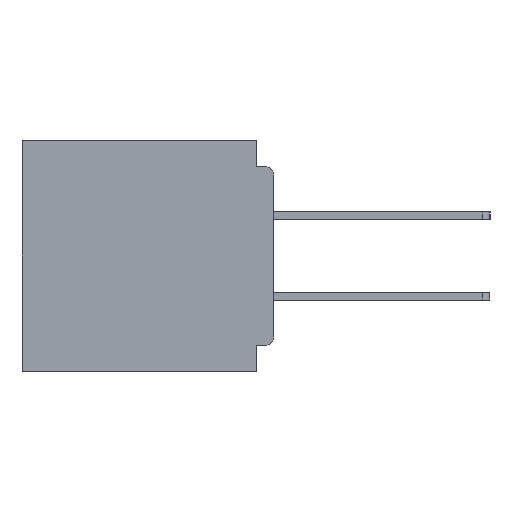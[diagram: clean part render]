
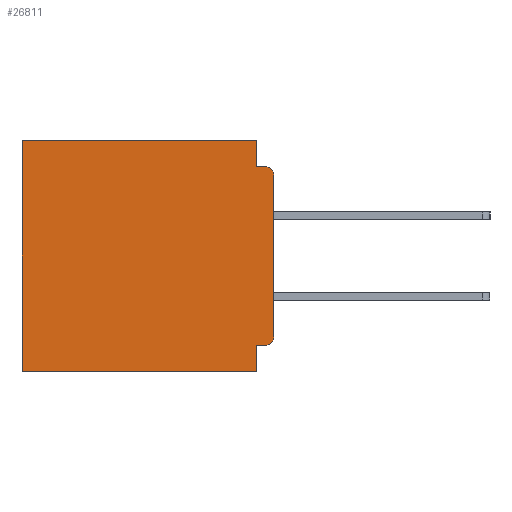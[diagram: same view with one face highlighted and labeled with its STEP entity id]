
A CAD part, left-side view. The second image highlights one B-rep face of the part: STEP entity #26811.
In plain terms, the highlighted planar face has unit normal (-1, 0, 0).
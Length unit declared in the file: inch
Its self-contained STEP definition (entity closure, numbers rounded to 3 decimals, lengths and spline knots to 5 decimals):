
#388 = CARTESIAN_POINT ( 'NONE',  ( 0.3, 0.031, 0. ) ) ;
#550 = CARTESIAN_POINT ( 'NONE',  ( 0.3, 0., -0.4 ) ) ;
#1070 = ORIENTED_EDGE ( 'NONE', *, *, #37587, .T. ) ;
#2581 = ORIENTED_EDGE ( 'NONE', *, *, #10394, .F. ) ;
#2887 = LINE ( 'NONE', #26888, #10167 ) ;
#3067 = ORIENTED_EDGE ( 'NONE', *, *, #6784, .F. ) ;
#3721 = DIRECTION ( 'NONE',  ( 1., 0., 0. ) ) ;
#3851 = CARTESIAN_POINT ( 'NONE',  ( 0.3, 0.437, 0. ) ) ;
#3932 = VECTOR ( 'NONE', #30655, 39.37008 ) ;
#4129 = VERTEX_POINT ( 'NONE', #21061 ) ;
#4271 = EDGE_CURVE ( 'NONE', #32339, #22659, #35562, .T. ) ;
#4812 = CARTESIAN_POINT ( 'NONE',  ( 0.3, 0., -0.045 ) ) ;
#4949 = VERTEX_POINT ( 'NONE', #7442 ) ;
#5126 = CARTESIAN_POINT ( 'NONE',  ( 0.3, 0., 0. ) ) ;
#5230 = ORIENTED_EDGE ( 'NONE', *, *, #27300, .T. ) ;
#5652 = AXIS2_PLACEMENT_3D ( 'NONE', #24552, #6122, #27612 ) ;
#6122 = DIRECTION ( 'NONE',  ( -1., 0., 0. ) ) ;
#6219 = AXIS2_PLACEMENT_3D ( 'NONE', #30311, #11955, #33346 ) ;
#6582 = EDGE_CURVE ( 'NONE', #6972, #24059, #34110, .T. ) ;
#6784 = EDGE_CURVE ( 'NONE', #4949, #7276, #2887, .T. ) ;
#6972 = VERTEX_POINT ( 'NONE', #37114 ) ;
#7069 = CIRCLE ( 'NONE', #5652, 0.015 ) ;
#7276 = VERTEX_POINT ( 'NONE', #20208 ) ;
#7338 = ORIENTED_EDGE ( 'NONE', *, *, #4271, .T. ) ;
#7442 = CARTESIAN_POINT ( 'NONE',  ( 0.3, 0., -0.06 ) ) ;
#7525 = VECTOR ( 'NONE', #17729, 39.37008 ) ;
#7939 = DIRECTION ( 'NONE',  ( 0., -1., 0. ) ) ;
#8235 = ORIENTED_EDGE ( 'NONE', *, *, #6582, .F. ) ;
#8476 = VECTOR ( 'NONE', #7939, 39.37008 ) ;
#8513 = DIRECTION ( 'NONE',  ( 0., 0., -1. ) ) ;
#9272 = AXIS2_PLACEMENT_3D ( 'NONE', #550, #3721, #25249 ) ;
#9529 = CARTESIAN_POINT ( 'NONE',  ( 0.3, 0., -0.355 ) ) ;
#9587 = DIRECTION ( 'NONE',  ( 0., 0., -1. ) ) ;
#9602 = DIRECTION ( 'NONE',  ( 0., 1., 0. ) ) ;
#10167 = VECTOR ( 'NONE', #8513, 39.37008 ) ;
#10394 = EDGE_CURVE ( 'NONE', #36185, #4129, #24817, .T. ) ;
#10654 = VECTOR ( 'NONE', #29050, 39.37008 ) ;
#10665 = CARTESIAN_POINT ( 'NONE',  ( 0.3, 0.031, -0.4 ) ) ;
#11060 = CARTESIAN_POINT ( 'NONE',  ( 0.3, 0.031, -0.045 ) ) ;
#11415 = VERTEX_POINT ( 'NONE', #19055 ) ;
#11955 = DIRECTION ( 'NONE',  ( -1., 0., 0. ) ) ;
#12642 = DIRECTION ( 'NONE',  ( 0., 1., 0. ) ) ;
#12703 = CARTESIAN_POINT ( 'NONE',  ( 0.3, 0.437, -0.4 ) ) ;
#14266 = ORIENTED_EDGE ( 'NONE', *, *, #19212, .F. ) ;
#15522 = CARTESIAN_POINT ( 'NONE',  ( 0.3, 0.031, -0.4 ) ) ;
#15609 = EDGE_CURVE ( 'NONE', #32339, #36185, #31038, .T. ) ;
#15971 = ORIENTED_EDGE ( 'NONE', *, *, #29117, .T. ) ;
#16676 = ORIENTED_EDGE ( 'NONE', *, *, #15609, .F. ) ;
#17729 = DIRECTION ( 'NONE',  ( 0., 0., -1. ) ) ;
#18768 = CARTESIAN_POINT ( 'NONE',  ( 0.3, 0.437, -0.4 ) ) ;
#18920 = CARTESIAN_POINT ( 'NONE',  ( 0.3, 0., -0.4 ) ) ;
#19055 = CARTESIAN_POINT ( 'NONE',  ( 0.3, 0.015, -0.355 ) ) ;
#19136 = PLANE ( 'NONE',  #9272 ) ;
#19212 = EDGE_CURVE ( 'NONE', #24059, #19216, #27906, .T. ) ;
#19216 = VERTEX_POINT ( 'NONE', #12703 ) ;
#19486 = VECTOR ( 'NONE', #9587, 39.37008 ) ;
#20208 = CARTESIAN_POINT ( 'NONE',  ( 0.3, 0., -0.34 ) ) ;
#20551 = VECTOR ( 'NONE', #12642, 39.37008 ) ;
#21061 = CARTESIAN_POINT ( 'NONE',  ( 0.3, 0.015, -0.045 ) ) ;
#22254 = EDGE_LOOP ( 'NONE', ( #3067, #1070, #2581, #16676, #7338, #15971, #14266, #8235, #24035, #5230 ) ) ;
#22659 = VERTEX_POINT ( 'NONE', #3851 ) ;
#24035 = ORIENTED_EDGE ( 'NONE', *, *, #37718, .F. ) ;
#24059 = VERTEX_POINT ( 'NONE', #15522 ) ;
#24552 = CARTESIAN_POINT ( 'NONE',  ( 0.3, 0.015, -0.34 ) ) ;
#24817 = LINE ( 'NONE', #4812, #8476 ) ;
#25249 = DIRECTION ( 'NONE',  ( 0., 0., -1. ) ) ;
#26232 = CIRCLE ( 'NONE', #6219, 0.015 ) ;
#26811 = ADVANCED_FACE ( 'NONE', ( #29673 ), #19136, .F. ) ;
#26888 = CARTESIAN_POINT ( 'NONE',  ( 0.3, 0., -0.4 ) ) ;
#26947 = VECTOR ( 'NONE', #9602, 39.37008 ) ;
#27300 = EDGE_CURVE ( 'NONE', #11415, #7276, #7069, .T. ) ;
#27570 = LINE ( 'NONE', #18768, #19486 ) ;
#27612 = DIRECTION ( 'NONE',  ( 0., 0., -1. ) ) ;
#27906 = LINE ( 'NONE', #18920, #26947 ) ;
#29050 = DIRECTION ( 'NONE',  ( 0., 0., -1. ) ) ;
#29117 = EDGE_CURVE ( 'NONE', #22659, #19216, #27570, .T. ) ;
#29673 = FACE_OUTER_BOUND ( 'NONE', #22254, .T. ) ;
#30311 = CARTESIAN_POINT ( 'NONE',  ( 0.3, 0.015, -0.06 ) ) ;
#30655 = DIRECTION ( 'NONE',  ( 0., 1., 0. ) ) ;
#31038 = LINE ( 'NONE', #39018, #7525 ) ;
#32339 = VERTEX_POINT ( 'NONE', #388 ) ;
#33346 = DIRECTION ( 'NONE',  ( 0., 0., -1. ) ) ;
#34110 = LINE ( 'NONE', #10665, #10654 ) ;
#35562 = LINE ( 'NONE', #5126, #3932 ) ;
#36185 = VERTEX_POINT ( 'NONE', #11060 ) ;
#36699 = LINE ( 'NONE', #9529, #20551 ) ;
#37114 = CARTESIAN_POINT ( 'NONE',  ( 0.3, 0.031, -0.355 ) ) ;
#37587 = EDGE_CURVE ( 'NONE', #4949, #4129, #26232, .T. ) ;
#37718 = EDGE_CURVE ( 'NONE', #11415, #6972, #36699, .T. ) ;
#39018 = CARTESIAN_POINT ( 'NONE',  ( 0.3, 0.031, 0. ) ) ;
